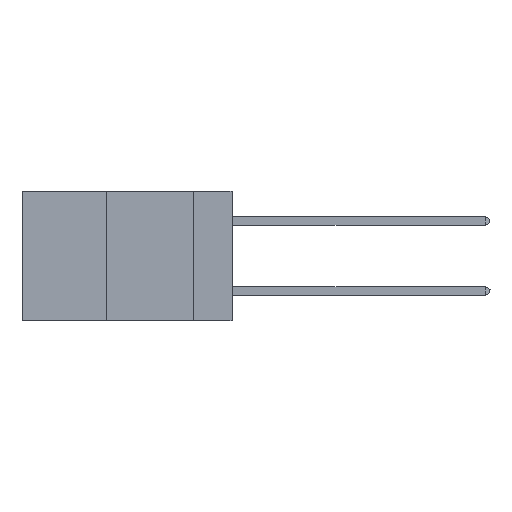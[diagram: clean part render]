
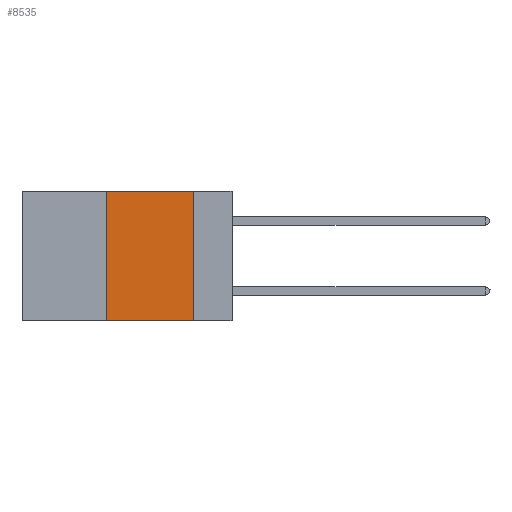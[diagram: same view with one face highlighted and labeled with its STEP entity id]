
A CAD part, left-side view. The second image highlights one B-rep face of the part: STEP entity #8535.
In plain terms, the highlighted planar face has unit normal (-1, 0, 0).
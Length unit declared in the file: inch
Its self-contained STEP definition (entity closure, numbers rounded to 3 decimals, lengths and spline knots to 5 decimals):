
#357 = CARTESIAN_POINT ( 'NONE',  ( 0., 0.6, -0.37 ) ) ;
#610 = CARTESIAN_POINT ( 'NONE',  ( 0., 0.36, 0. ) ) ;
#1044 = EDGE_CURVE ( 'NONE', #11431, #11743, #10499, .T. ) ;
#1054 = FACE_OUTER_BOUND ( 'NONE', #5799, .T. ) ;
#1657 = DIRECTION ( 'NONE',  ( 0., 0., -1. ) ) ;
#1663 = CARTESIAN_POINT ( 'NONE',  ( 0., 0.36, -0.37 ) ) ;
#1860 = EDGE_CURVE ( 'NONE', #12168, #11743, #2604, .T. ) ;
#2604 = LINE ( 'NONE', #11470, #9027 ) ;
#2789 = DIRECTION ( 'NONE',  ( 1., 0., 0. ) ) ;
#3624 = ORIENTED_EDGE ( 'NONE', *, *, #6742, .F. ) ;
#4336 = VERTEX_POINT ( 'NONE', #610 ) ;
#5293 = EDGE_CURVE ( 'NONE', #4336, #12168, #7961, .T. ) ;
#5720 = ORIENTED_EDGE ( 'NONE', *, *, #5293, .F. ) ;
#5799 = EDGE_LOOP ( 'NONE', ( #13164, #5720, #3624, #13161 ) ) ;
#5946 = LINE ( 'NONE', #10263, #8020 ) ;
#6742 = EDGE_CURVE ( 'NONE', #11431, #4336, #5946, .T. ) ;
#7606 = VECTOR ( 'NONE', #8571, 39.37008 ) ;
#7817 = PLANE ( 'NONE',  #12407 ) ;
#7961 = LINE ( 'NONE', #8983, #12951 ) ;
#8020 = VECTOR ( 'NONE', #12351, 39.37008 ) ;
#8535 = ADVANCED_FACE ( 'NONE', ( #1054 ), #7817, .F. ) ;
#8571 = DIRECTION ( 'NONE',  ( 0., -1., 0. ) ) ;
#8827 = CARTESIAN_POINT ( 'NONE',  ( 0., 0.6, 0. ) ) ;
#8983 = CARTESIAN_POINT ( 'NONE',  ( 0., 0.6, 0. ) ) ;
#9027 = VECTOR ( 'NONE', #9517, 39.37008 ) ;
#9517 = DIRECTION ( 'NONE',  ( 0., 0., -1. ) ) ;
#10263 = CARTESIAN_POINT ( 'NONE',  ( 0., 0.36, 0. ) ) ;
#10499 = LINE ( 'NONE', #357, #7606 ) ;
#10520 = CARTESIAN_POINT ( 'NONE',  ( 0., 0.11, -0.37 ) ) ;
#10980 = DIRECTION ( 'NONE',  ( 0., -1., 0. ) ) ;
#11431 = VERTEX_POINT ( 'NONE', #1663 ) ;
#11470 = CARTESIAN_POINT ( 'NONE',  ( 0., 0.11, 0. ) ) ;
#11743 = VERTEX_POINT ( 'NONE', #10520 ) ;
#12135 = CARTESIAN_POINT ( 'NONE',  ( 0., 0.11, 0. ) ) ;
#12168 = VERTEX_POINT ( 'NONE', #12135 ) ;
#12351 = DIRECTION ( 'NONE',  ( 0., 0., 1. ) ) ;
#12407 = AXIS2_PLACEMENT_3D ( 'NONE', #8827, #2789, #1657 ) ;
#12951 = VECTOR ( 'NONE', #10980, 39.37008 ) ;
#13161 = ORIENTED_EDGE ( 'NONE', *, *, #1044, .T. ) ;
#13164 = ORIENTED_EDGE ( 'NONE', *, *, #1860, .F. ) ;
